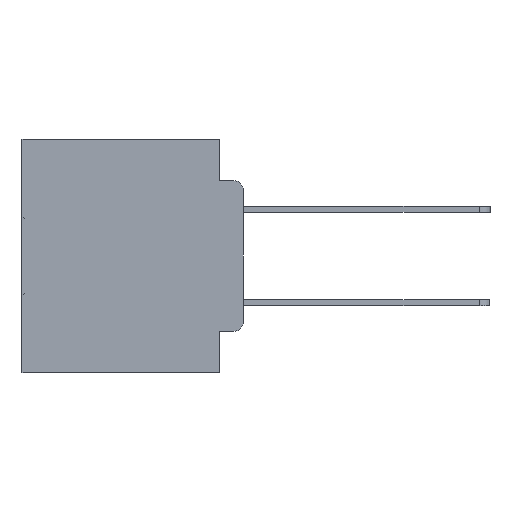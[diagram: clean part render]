
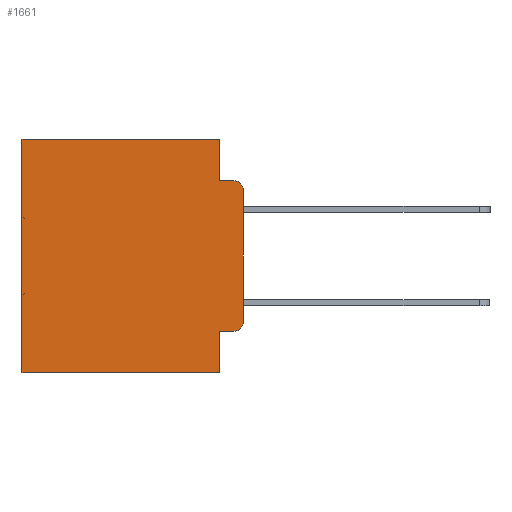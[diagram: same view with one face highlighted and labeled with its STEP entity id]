
A CAD part, left-side view. The second image highlights one B-rep face of the part: STEP entity #1661.
In plain terms, the highlighted planar face has unit normal (-1, 0, 0).
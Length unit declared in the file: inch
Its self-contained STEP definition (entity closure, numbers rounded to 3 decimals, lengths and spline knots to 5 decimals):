
#338 = EDGE_CURVE ( 'NONE', #19115, #10672, #32624, .T. ) ;
#737 = LINE ( 'NONE', #23623, #13877 ) ;
#938 = LINE ( 'NONE', #4868, #20115 ) ;
#953 = ORIENTED_EDGE ( 'NONE', *, *, #6664, .F. ) ;
#1281 = ORIENTED_EDGE ( 'NONE', *, *, #19518, .T. ) ;
#1661 = ADVANCED_FACE ( 'NONE', ( #19890 ), #33081, .F. ) ;
#2348 = ORIENTED_EDGE ( 'NONE', *, *, #338, .T. ) ;
#2606 = CARTESIAN_POINT ( 'NONE',  ( 0.298, 0.051, -0.4115 ) ) ;
#2655 = CARTESIAN_POINT ( 'NONE',  ( 0.298, 0.051, -0.0885 ) ) ;
#3042 = ORIENTED_EDGE ( 'NONE', *, *, #31559, .T. ) ;
#3819 = ORIENTED_EDGE ( 'NONE', *, *, #14362, .F. ) ;
#4095 = AXIS2_PLACEMENT_3D ( 'NONE', #25693, #25991, #25911 ) ;
#4492 = VECTOR ( 'NONE', #30254, 39.37008 ) ;
#4572 = ORIENTED_EDGE ( 'NONE', *, *, #5544, .T. ) ;
#4868 = CARTESIAN_POINT ( 'NONE',  ( 0.298, 0.051, -0.0885 ) ) ;
#5002 = ORIENTED_EDGE ( 'NONE', *, *, #22974, .F. ) ;
#5544 = EDGE_CURVE ( 'NONE', #12571, #12335, #23292, .T. ) ;
#5841 = VERTEX_POINT ( 'NONE', #2655 ) ;
#6010 = DIRECTION ( 'NONE',  ( 0., 0., -1. ) ) ;
#6561 = CARTESIAN_POINT ( 'NONE',  ( 0.298, 0.473, 0. ) ) ;
#6664 = EDGE_CURVE ( 'NONE', #16505, #12335, #32030, .T. ) ;
#7263 = ORIENTED_EDGE ( 'NONE', *, *, #10879, .T. ) ;
#7608 = VERTEX_POINT ( 'NONE', #16287 ) ;
#8094 = DIRECTION ( 'NONE',  ( 0., -1., 0. ) ) ;
#8183 = VECTOR ( 'NONE', #13821, 39.37008 ) ;
#8358 = LINE ( 'NONE', #13242, #21313 ) ;
#8445 = AXIS2_PLACEMENT_3D ( 'NONE', #13194, #14292, #12643 ) ;
#9275 = VECTOR ( 'NONE', #6010, 39.37008 ) ;
#9297 = CARTESIAN_POINT ( 'NONE',  ( 0.298, 0.051, -0.5 ) ) ;
#9481 = EDGE_CURVE ( 'NONE', #10539, #12472, #15135, .T. ) ;
#9661 = VECTOR ( 'NONE', #26202, 39.37008 ) ;
#9715 = LINE ( 'NONE', #6561, #22634 ) ;
#9748 = DIRECTION ( 'NONE',  ( -1., 0., 0. ) ) ;
#10194 = VERTEX_POINT ( 'NONE', #2606 ) ;
#10539 = VERTEX_POINT ( 'NONE', #9297 ) ;
#10672 = VERTEX_POINT ( 'NONE', #20137 ) ;
#10783 = CARTESIAN_POINT ( 'NONE',  ( 0.298, 0., -0.1085 ) ) ;
#10879 = EDGE_CURVE ( 'NONE', #10194, #12571, #737, .T. ) ;
#12335 = VERTEX_POINT ( 'NONE', #19582 ) ;
#12472 = VERTEX_POINT ( 'NONE', #30353 ) ;
#12571 = VERTEX_POINT ( 'NONE', #12810 ) ;
#12643 = DIRECTION ( 'NONE',  ( 0., 0., -1. ) ) ;
#12810 = CARTESIAN_POINT ( 'NONE',  ( 0.298, 0.02, -0.4115 ) ) ;
#13194 = CARTESIAN_POINT ( 'NONE',  ( 0.298, 0., 0. ) ) ;
#13242 = CARTESIAN_POINT ( 'NONE',  ( 0.298, 0.051, 0. ) ) ;
#13821 = DIRECTION ( 'NONE',  ( 0., 1., 0. ) ) ;
#13831 = CARTESIAN_POINT ( 'NONE',  ( 0.298, 0.051, 0. ) ) ;
#13877 = VECTOR ( 'NONE', #8094, 39.37008 ) ;
#14292 = DIRECTION ( 'NONE',  ( 1., 0., 0. ) ) ;
#14362 = EDGE_CURVE ( 'NONE', #10194, #10539, #8358, .T. ) ;
#15135 = LINE ( 'NONE', #26578, #8183 ) ;
#15825 = DIRECTION ( 'NONE',  ( 0., 0., -1. ) ) ;
#16287 = CARTESIAN_POINT ( 'NONE',  ( 0.298, 0.02, -0.0885 ) ) ;
#16505 = VERTEX_POINT ( 'NONE', #10783 ) ;
#19115 = VERTEX_POINT ( 'NONE', #23053 ) ;
#19350 = CARTESIAN_POINT ( 'NONE',  ( 0.298, 0., 0. ) ) ;
#19518 = EDGE_CURVE ( 'NONE', #10672, #12472, #9715, .T. ) ;
#19582 = CARTESIAN_POINT ( 'NONE',  ( 0.298, 0., -0.3915 ) ) ;
#19890 = FACE_OUTER_BOUND ( 'NONE', #20913, .T. ) ;
#20115 = VECTOR ( 'NONE', #20474, 39.37008 ) ;
#20137 = CARTESIAN_POINT ( 'NONE',  ( 0.298, 0.473, 0. ) ) ;
#20474 = DIRECTION ( 'NONE',  ( 0., -1., 0. ) ) ;
#20913 = EDGE_LOOP ( 'NONE', ( #953, #3042, #22997, #5002, #2348, #1281, #23532, #3819, #7263, #4572 ) ) ;
#21297 = AXIS2_PLACEMENT_3D ( 'NONE', #25241, #9748, #27798 ) ;
#21313 = VECTOR ( 'NONE', #15825, 39.37008 ) ;
#22634 = VECTOR ( 'NONE', #24620, 39.37008 ) ;
#22974 = EDGE_CURVE ( 'NONE', #19115, #5841, #29832, .T. ) ;
#22997 = ORIENTED_EDGE ( 'NONE', *, *, #28157, .F. ) ;
#23053 = CARTESIAN_POINT ( 'NONE',  ( 0.298, 0.051, 0. ) ) ;
#23292 = CIRCLE ( 'NONE', #4095, 0.02 ) ;
#23532 = ORIENTED_EDGE ( 'NONE', *, *, #9481, .F. ) ;
#23623 = CARTESIAN_POINT ( 'NONE',  ( 0.298, 0.051, -0.4115 ) ) ;
#24620 = DIRECTION ( 'NONE',  ( 0., 0., -1. ) ) ;
#25241 = CARTESIAN_POINT ( 'NONE',  ( 0.298, 0.02, -0.1085 ) ) ;
#25693 = CARTESIAN_POINT ( 'NONE',  ( 0.298, 0.02, -0.3915 ) ) ;
#25844 = CARTESIAN_POINT ( 'NONE',  ( 0.298, 0., 0. ) ) ;
#25911 = DIRECTION ( 'NONE',  ( 0., 0., -1. ) ) ;
#25991 = DIRECTION ( 'NONE',  ( -1., 0., 0. ) ) ;
#26202 = DIRECTION ( 'NONE',  ( 0., 1., 0. ) ) ;
#26578 = CARTESIAN_POINT ( 'NONE',  ( 0.298, 0., -0.5 ) ) ;
#27798 = DIRECTION ( 'NONE',  ( 0., 0., -1. ) ) ;
#28157 = EDGE_CURVE ( 'NONE', #5841, #7608, #938, .T. ) ;
#29832 = LINE ( 'NONE', #13831, #9275 ) ;
#30254 = DIRECTION ( 'NONE',  ( 0., 0., -1. ) ) ;
#30353 = CARTESIAN_POINT ( 'NONE',  ( 0.298, 0.473, -0.5 ) ) ;
#31132 = CIRCLE ( 'NONE', #21297, 0.02 ) ;
#31559 = EDGE_CURVE ( 'NONE', #16505, #7608, #31132, .T. ) ;
#32030 = LINE ( 'NONE', #25844, #4492 ) ;
#32624 = LINE ( 'NONE', #19350, #9661 ) ;
#33081 = PLANE ( 'NONE',  #8445 ) ;
